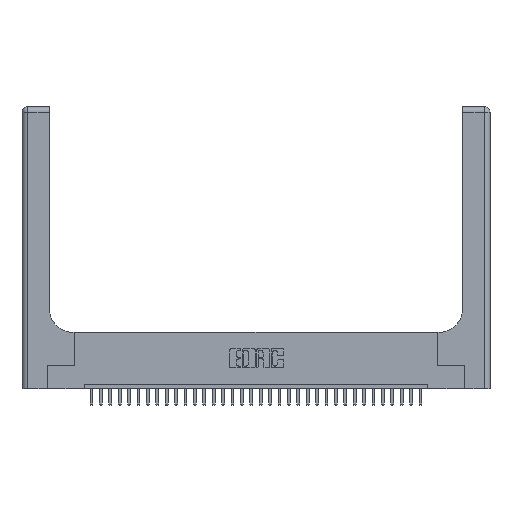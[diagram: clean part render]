
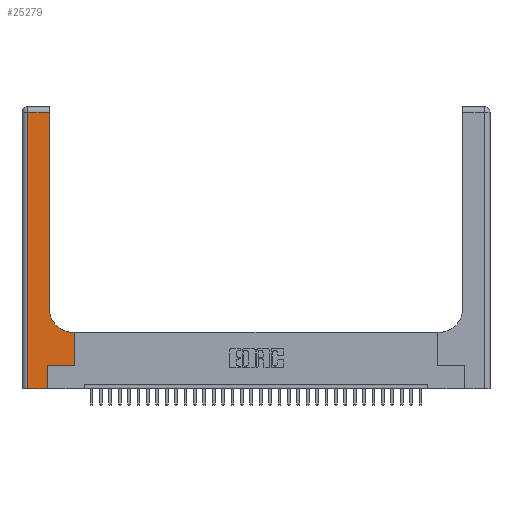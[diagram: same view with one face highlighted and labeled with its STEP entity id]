
A CAD part, top view. The second image highlights one B-rep face of the part: STEP entity #25279.
In plain terms, the highlighted planar face has unit normal (0, 0, 1).
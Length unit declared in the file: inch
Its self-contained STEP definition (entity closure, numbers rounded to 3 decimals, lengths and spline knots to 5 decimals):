
#27 = EDGE_LOOP ( 'NONE', ( #28549, #6642, #16477, #15248, #14080, #29650, #8797, #30530, #12695 ) ) ;
#1537 = DIRECTION ( 'NONE',  ( -1., 0., 0. ) ) ;
#1540 = CARTESIAN_POINT ( 'NONE',  ( 0.06, 3., 0.37 ) ) ;
#1614 = VERTEX_POINT ( 'NONE', #17857 ) ;
#2082 = DIRECTION ( 'NONE',  ( 0., 0., -1. ) ) ;
#2120 = FACE_OUTER_BOUND ( 'NONE', #27, .T. ) ;
#2272 = CARTESIAN_POINT ( 'NONE',  ( 0.5585, 0.25, 0.37 ) ) ;
#2397 = CARTESIAN_POINT ( 'NONE',  ( 0.2915, 0.85, 0.37 ) ) ;
#2666 = EDGE_CURVE ( 'NONE', #23590, #15386, #28669, .T. ) ;
#3110 = CARTESIAN_POINT ( 'NONE',  ( 0.06, 2.94, 0.37 ) ) ;
#3474 = DIRECTION ( 'NONE',  ( 0., 1., 0. ) ) ;
#4092 = VERTEX_POINT ( 'NONE', #31985 ) ;
#4671 = DIRECTION ( 'NONE',  ( -1., 0., 0. ) ) ;
#5546 = LINE ( 'NONE', #13911, #12048 ) ;
#6571 = CARTESIAN_POINT ( 'NONE',  ( 0., 0., 0.37 ) ) ;
#6642 = ORIENTED_EDGE ( 'NONE', *, *, #13509, .T. ) ;
#7184 = VECTOR ( 'NONE', #15242, 39.37008 ) ;
#7268 = DIRECTION ( 'NONE',  ( 1., 0., 0. ) ) ;
#8017 = VERTEX_POINT ( 'NONE', #26091 ) ;
#8797 = ORIENTED_EDGE ( 'NONE', *, *, #30350, .T. ) ;
#8933 = VERTEX_POINT ( 'NONE', #24848 ) ;
#9068 = EDGE_CURVE ( 'NONE', #4092, #8933, #5546, .T. ) ;
#9140 = VECTOR ( 'NONE', #3474, 39.37008 ) ;
#9442 = CARTESIAN_POINT ( 'NONE',  ( 0.2915, 0.6, 0.37 ) ) ;
#9580 = LINE ( 'NONE', #27695, #24009 ) ;
#9612 = AXIS2_PLACEMENT_3D ( 'NONE', #12350, #2082, #7268 ) ;
#9939 = EDGE_CURVE ( 'NONE', #15386, #8017, #29550, .T. ) ;
#10919 = EDGE_CURVE ( 'NONE', #20450, #23823, #24370, .T. ) ;
#11040 = CARTESIAN_POINT ( 'NONE',  ( 0., 3., 0.37 ) ) ;
#11505 = CARTESIAN_POINT ( 'NONE',  ( 0.2915, 3., 0.37 ) ) ;
#12048 = VECTOR ( 'NONE', #18808, 39.37008 ) ;
#12350 = CARTESIAN_POINT ( 'NONE',  ( 0.5415, 0.85, 0.37 ) ) ;
#12695 = ORIENTED_EDGE ( 'NONE', *, *, #2666, .T. ) ;
#12990 = VECTOR ( 'NONE', #24872, 39.37008 ) ;
#13509 = EDGE_CURVE ( 'NONE', #8017, #20450, #9580, .T. ) ;
#13783 = LINE ( 'NONE', #6571, #12990 ) ;
#13911 = CARTESIAN_POINT ( 'NONE',  ( 0.269, 0., 0.37 ) ) ;
#13984 = DIRECTION ( 'NONE',  ( 1., 0., 0. ) ) ;
#14004 = CARTESIAN_POINT ( 'NONE',  ( 0.5585, 0.6, 0.37 ) ) ;
#14080 = ORIENTED_EDGE ( 'NONE', *, *, #9068, .T. ) ;
#15242 = DIRECTION ( 'NONE',  ( 0., 1., 0. ) ) ;
#15248 = ORIENTED_EDGE ( 'NONE', *, *, #27739, .T. ) ;
#15386 = VERTEX_POINT ( 'NONE', #2397 ) ;
#15526 = VERTEX_POINT ( 'NONE', #14004 ) ;
#16477 = ORIENTED_EDGE ( 'NONE', *, *, #10919, .T. ) ;
#17857 = CARTESIAN_POINT ( 'NONE',  ( 0.5585, 0.25, 0.37 ) ) ;
#18092 = CARTESIAN_POINT ( 'NONE',  ( 0.5415, 0.6, 0.37 ) ) ;
#18808 = DIRECTION ( 'NONE',  ( 0., 1., 0. ) ) ;
#19019 = CARTESIAN_POINT ( 'NONE',  ( 0.06, 0., 0.37 ) ) ;
#19118 = VECTOR ( 'NONE', #1537, 39.37008 ) ;
#20450 = VERTEX_POINT ( 'NONE', #3110 ) ;
#21593 = CARTESIAN_POINT ( 'NONE',  ( 0.269, 0.25, 0.37 ) ) ;
#23219 = LINE ( 'NONE', #2272, #7184 ) ;
#23590 = VERTEX_POINT ( 'NONE', #18092 ) ;
#23823 = VERTEX_POINT ( 'NONE', #19019 ) ;
#24009 = VECTOR ( 'NONE', #4671, 39.37008 ) ;
#24370 = LINE ( 'NONE', #1540, #26773 ) ;
#24848 = CARTESIAN_POINT ( 'NONE',  ( 0.269, 0.25, 0.37 ) ) ;
#24872 = DIRECTION ( 'NONE',  ( 1., 0., 0. ) ) ;
#25251 = EDGE_CURVE ( 'NONE', #8933, #1614, #26609, .T. ) ;
#25279 = ADVANCED_FACE ( 'NONE', ( #2120 ), #26402, .F. ) ;
#25441 = VECTOR ( 'NONE', #13984, 39.37008 ) ;
#25925 = LINE ( 'NONE', #9442, #19118 ) ;
#26091 = CARTESIAN_POINT ( 'NONE',  ( 0.2915, 2.94, 0.37 ) ) ;
#26107 = EDGE_CURVE ( 'NONE', #15526, #23590, #25925, .T. ) ;
#26402 = PLANE ( 'NONE',  #29059 ) ;
#26609 = LINE ( 'NONE', #21593, #25441 ) ;
#26773 = VECTOR ( 'NONE', #32593, 39.37008 ) ;
#27695 = CARTESIAN_POINT ( 'NONE',  ( 0., 2.94, 0.37 ) ) ;
#27739 = EDGE_CURVE ( 'NONE', #23823, #4092, #13783, .T. ) ;
#28549 = ORIENTED_EDGE ( 'NONE', *, *, #9939, .T. ) ;
#28669 = CIRCLE ( 'NONE', #9612, 0.25 ) ;
#28938 = DIRECTION ( 'NONE',  ( 0., 0., -1. ) ) ;
#29059 = AXIS2_PLACEMENT_3D ( 'NONE', #11040, #28938, #31488 ) ;
#29550 = LINE ( 'NONE', #11505, #9140 ) ;
#29650 = ORIENTED_EDGE ( 'NONE', *, *, #25251, .T. ) ;
#30350 = EDGE_CURVE ( 'NONE', #1614, #15526, #23219, .T. ) ;
#30530 = ORIENTED_EDGE ( 'NONE', *, *, #26107, .T. ) ;
#31488 = DIRECTION ( 'NONE',  ( -1., 0., 0. ) ) ;
#31985 = CARTESIAN_POINT ( 'NONE',  ( 0.269, 0., 0.37 ) ) ;
#32593 = DIRECTION ( 'NONE',  ( 0., -1., 0. ) ) ;
